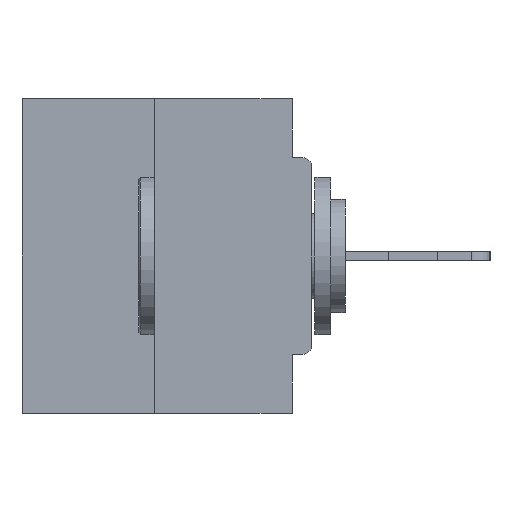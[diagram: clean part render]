
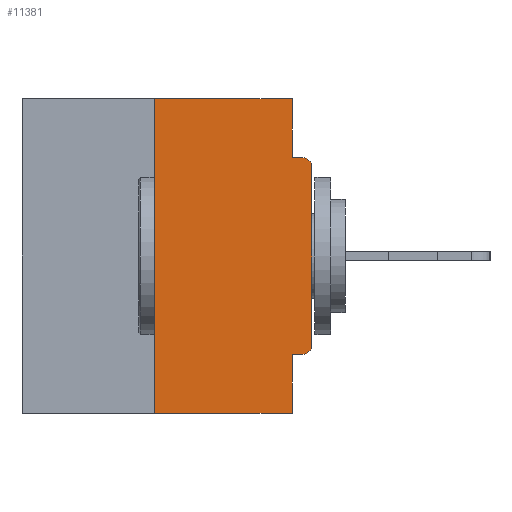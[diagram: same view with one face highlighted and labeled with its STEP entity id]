
A CAD part, left-side view. The second image highlights one B-rep face of the part: STEP entity #11381.
In plain terms, the highlighted planar face has unit normal (-1, 0, 0).
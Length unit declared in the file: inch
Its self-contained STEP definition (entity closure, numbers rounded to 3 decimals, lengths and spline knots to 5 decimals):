
#73 = EDGE_CURVE ( 'NONE', #12059, #15067, #25200, .T. ) ;
#978 = VECTOR ( 'NONE', #5802, 39.37008 ) ;
#2056 = EDGE_CURVE ( 'NONE', #10630, #6802, #32975, .T. ) ;
#2255 = DIRECTION ( 'NONE',  ( 0., 1., 0. ) ) ;
#2260 = ORIENTED_EDGE ( 'NONE', *, *, #18215, .F. ) ;
#3091 = DIRECTION ( 'NONE',  ( 0., 0., -1. ) ) ;
#3751 = ORIENTED_EDGE ( 'NONE', *, *, #2056, .F. ) ;
#3802 = LINE ( 'NONE', #26571, #18728 ) ;
#4673 = CARTESIAN_POINT ( 'NONE',  ( 0., 0., -0.1085 ) ) ;
#4791 = DIRECTION ( 'NONE',  ( 1., 0., 0. ) ) ;
#4936 = LINE ( 'NONE', #32302, #38715 ) ;
#5264 = VECTOR ( 'NONE', #7598, 39.37008 ) ;
#5802 = DIRECTION ( 'NONE',  ( 0., -1., 0. ) ) ;
#6168 = VERTEX_POINT ( 'NONE', #4673 ) ;
#6774 = ORIENTED_EDGE ( 'NONE', *, *, #32288, .F. ) ;
#6802 = VERTEX_POINT ( 'NONE', #28325 ) ;
#7362 = AXIS2_PLACEMENT_3D ( 'NONE', #33301, #4791, #27073 ) ;
#7598 = DIRECTION ( 'NONE',  ( 0., 0., 1. ) ) ;
#7635 = VERTEX_POINT ( 'NONE', #26172 ) ;
#7791 = ORIENTED_EDGE ( 'NONE', *, *, #37616, .T. ) ;
#8176 = FACE_OUTER_BOUND ( 'NONE', #8283, .T. ) ;
#8283 = EDGE_LOOP ( 'NONE', ( #27180, #3751, #30168, #22658, #6774, #7791, #24697, #18211, #2260, #20204 ) ) ;
#8776 = CARTESIAN_POINT ( 'NONE',  ( 0., 0.46, -0.5 ) ) ;
#8829 = CIRCLE ( 'NONE', #22724, 0.015 ) ;
#9624 = LINE ( 'NONE', #14829, #39333 ) ;
#9835 = AXIS2_PLACEMENT_3D ( 'NONE', #30470, #11467, #33655 ) ;
#9868 = DIRECTION ( 'NONE',  ( 0., 0., 1. ) ) ;
#9887 = EDGE_CURVE ( 'NONE', #6168, #38339, #8829, .T. ) ;
#10630 = VERTEX_POINT ( 'NONE', #11174 ) ;
#10750 = DIRECTION ( 'NONE',  ( 0., -1., 0. ) ) ;
#11174 = CARTESIAN_POINT ( 'NONE',  ( 0., 0.25, -0.5 ) ) ;
#11381 = ADVANCED_FACE ( 'NONE', ( #8176 ), #14289, .F. ) ;
#11467 = DIRECTION ( 'NONE',  ( -1., 0., 0. ) ) ;
#11880 = VERTEX_POINT ( 'NONE', #23115 ) ;
#12059 = VERTEX_POINT ( 'NONE', #14509 ) ;
#12713 = VERTEX_POINT ( 'NONE', #17636 ) ;
#12853 = EDGE_CURVE ( 'NONE', #10630, #11880, #17958, .T. ) ;
#13765 = LINE ( 'NONE', #20215, #5264 ) ;
#14289 = PLANE ( 'NONE',  #7362 ) ;
#14509 = CARTESIAN_POINT ( 'NONE',  ( 0., 0.031, 0. ) ) ;
#14829 = CARTESIAN_POINT ( 'NONE',  ( 0., 0.031, -0.5 ) ) ;
#15067 = VERTEX_POINT ( 'NONE', #22741 ) ;
#16193 = CARTESIAN_POINT ( 'NONE',  ( 0., 0.015, -0.1085 ) ) ;
#16276 = VERTEX_POINT ( 'NONE', #28524 ) ;
#17636 = CARTESIAN_POINT ( 'NONE',  ( 0., 0.031, -0.4065 ) ) ;
#17958 = LINE ( 'NONE', #8776, #978 ) ;
#18211 = ORIENTED_EDGE ( 'NONE', *, *, #9887, .T. ) ;
#18215 = EDGE_CURVE ( 'NONE', #15067, #38339, #4936, .T. ) ;
#18728 = VECTOR ( 'NONE', #10750, 39.37008 ) ;
#19337 = DIRECTION ( 'NONE',  ( 0., 0., -1. ) ) ;
#20191 = EDGE_CURVE ( 'NONE', #7635, #6168, #13765, .T. ) ;
#20204 = ORIENTED_EDGE ( 'NONE', *, *, #73, .F. ) ;
#20215 = CARTESIAN_POINT ( 'NONE',  ( 0., 0., 0. ) ) ;
#20827 = VECTOR ( 'NONE', #2255, 39.37008 ) ;
#22658 = ORIENTED_EDGE ( 'NONE', *, *, #37083, .F. ) ;
#22724 = AXIS2_PLACEMENT_3D ( 'NONE', #16193, #38364, #19337 ) ;
#22741 = CARTESIAN_POINT ( 'NONE',  ( 0., 0.031, -0.0935 ) ) ;
#22834 = DIRECTION ( 'NONE',  ( 0., -1., 0. ) ) ;
#23115 = CARTESIAN_POINT ( 'NONE',  ( 0., 0.031, -0.5 ) ) ;
#23841 = EDGE_CURVE ( 'NONE', #6802, #12059, #3802, .T. ) ;
#24554 = CARTESIAN_POINT ( 'NONE',  ( 0., 0., -0.4065 ) ) ;
#24697 = ORIENTED_EDGE ( 'NONE', *, *, #20191, .T. ) ;
#25200 = LINE ( 'NONE', #27484, #31647 ) ;
#25934 = CIRCLE ( 'NONE', #9835, 0.015 ) ;
#26172 = CARTESIAN_POINT ( 'NONE',  ( 0., 0., -0.3915 ) ) ;
#26571 = CARTESIAN_POINT ( 'NONE',  ( 0., 0.46, 0. ) ) ;
#27073 = DIRECTION ( 'NONE',  ( 0., 0., -1. ) ) ;
#27180 = ORIENTED_EDGE ( 'NONE', *, *, #23841, .F. ) ;
#27484 = CARTESIAN_POINT ( 'NONE',  ( 0., 0.031, 0. ) ) ;
#28325 = CARTESIAN_POINT ( 'NONE',  ( 0., 0.25, 0. ) ) ;
#28328 = CARTESIAN_POINT ( 'NONE',  ( 0., 0.25, 0. ) ) ;
#28524 = CARTESIAN_POINT ( 'NONE',  ( 0., 0.015, -0.4065 ) ) ;
#30168 = ORIENTED_EDGE ( 'NONE', *, *, #12853, .T. ) ;
#30470 = CARTESIAN_POINT ( 'NONE',  ( 0., 0.015, -0.3915 ) ) ;
#31647 = VECTOR ( 'NONE', #3091, 39.37008 ) ;
#31956 = VECTOR ( 'NONE', #9868, 39.37008 ) ;
#32288 = EDGE_CURVE ( 'NONE', #16276, #12713, #38657, .T. ) ;
#32302 = CARTESIAN_POINT ( 'NONE',  ( 0., 0., -0.0935 ) ) ;
#32975 = LINE ( 'NONE', #28328, #31956 ) ;
#33301 = CARTESIAN_POINT ( 'NONE',  ( 0., 0.46, 0. ) ) ;
#33655 = DIRECTION ( 'NONE',  ( 0., 0., -1. ) ) ;
#33847 = DIRECTION ( 'NONE',  ( 0., 0., -1. ) ) ;
#37083 = EDGE_CURVE ( 'NONE', #12713, #11880, #9624, .T. ) ;
#37616 = EDGE_CURVE ( 'NONE', #16276, #7635, #25934, .T. ) ;
#37860 = CARTESIAN_POINT ( 'NONE',  ( 0., 0.015, -0.0935 ) ) ;
#38339 = VERTEX_POINT ( 'NONE', #37860 ) ;
#38364 = DIRECTION ( 'NONE',  ( -1., 0., 0. ) ) ;
#38657 = LINE ( 'NONE', #24554, #20827 ) ;
#38715 = VECTOR ( 'NONE', #22834, 39.37008 ) ;
#39333 = VECTOR ( 'NONE', #33847, 39.37008 ) ;
